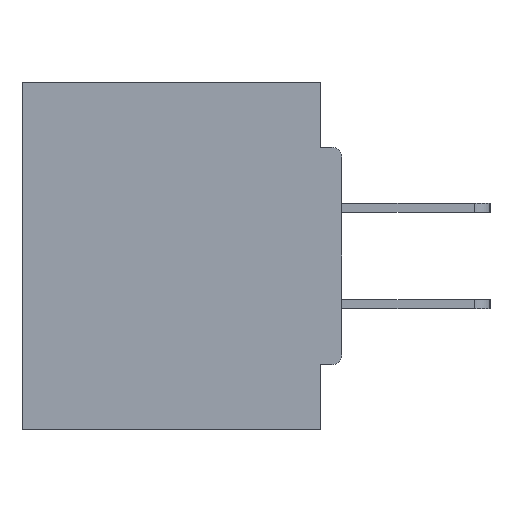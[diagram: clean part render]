
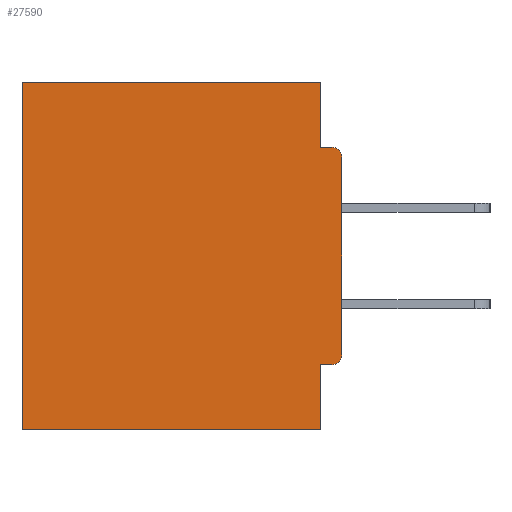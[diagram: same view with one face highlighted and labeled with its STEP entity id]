
A CAD part, left-side view. The second image highlights one B-rep face of the part: STEP entity #27590.
In plain terms, the highlighted planar face has unit normal (-1, 0, 0).
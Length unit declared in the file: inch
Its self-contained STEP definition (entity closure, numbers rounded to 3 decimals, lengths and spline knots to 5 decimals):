
#1164 = CIRCLE ( 'NONE', #3589, 0.015 ) ;
#1298 = CARTESIAN_POINT ( 'NONE',  ( 0.298, 0.031, -0.5 ) ) ;
#2060 = VECTOR ( 'NONE', #28027, 39.37008 ) ;
#2228 = CARTESIAN_POINT ( 'NONE',  ( 0.298, 0.031, -0.5 ) ) ;
#2380 = ORIENTED_EDGE ( 'NONE', *, *, #32719, .F. ) ;
#2655 = EDGE_CURVE ( 'NONE', #3849, #28235, #35394, .T. ) ;
#2682 = CARTESIAN_POINT ( 'NONE',  ( 0.298, 0.015, -0.4065 ) ) ;
#3080 = LINE ( 'NONE', #7466, #18006 ) ;
#3131 = DIRECTION ( 'NONE',  ( 0., 0., -1. ) ) ;
#3264 = CARTESIAN_POINT ( 'NONE',  ( 0.298, 0.015, -0.3915 ) ) ;
#3558 = EDGE_CURVE ( 'NONE', #12391, #12726, #29469, .T. ) ;
#3589 = AXIS2_PLACEMENT_3D ( 'NONE', #14710, #26165, #3684 ) ;
#3684 = DIRECTION ( 'NONE',  ( 0., 0., -1. ) ) ;
#3849 = VERTEX_POINT ( 'NONE', #35695 ) ;
#4348 = CARTESIAN_POINT ( 'NONE',  ( 0.298, 0.46, 0. ) ) ;
#5256 = DIRECTION ( 'NONE',  ( 0., 1., 0. ) ) ;
#6180 = DIRECTION ( 'NONE',  ( 0., 0., -1. ) ) ;
#7466 = CARTESIAN_POINT ( 'NONE',  ( 0.298, 0., -0.5 ) ) ;
#8186 = DIRECTION ( 'NONE',  ( 0., -1., 0. ) ) ;
#8608 = CARTESIAN_POINT ( 'NONE',  ( 0.298, 0.031, -0.5 ) ) ;
#9633 = CARTESIAN_POINT ( 'NONE',  ( 0.298, 0., -0.1085 ) ) ;
#10386 = LINE ( 'NONE', #34632, #16552 ) ;
#10844 = VERTEX_POINT ( 'NONE', #9633 ) ;
#11154 = EDGE_CURVE ( 'NONE', #19791, #27602, #3080, .T. ) ;
#11939 = CARTESIAN_POINT ( 'NONE',  ( 0.298, 0.46, -0.5 ) ) ;
#12018 = DIRECTION ( 'NONE',  ( 0., 1., 0. ) ) ;
#12109 = ORIENTED_EDGE ( 'NONE', *, *, #14190, .F. ) ;
#12391 = VERTEX_POINT ( 'NONE', #35027 ) ;
#12726 = VERTEX_POINT ( 'NONE', #15777 ) ;
#13450 = CARTESIAN_POINT ( 'NONE',  ( 0.298, 0.031, -0.4065 ) ) ;
#13462 = EDGE_CURVE ( 'NONE', #21836, #19791, #30617, .T. ) ;
#13523 = EDGE_CURVE ( 'NONE', #10844, #14720, #10386, .T. ) ;
#14168 = EDGE_CURVE ( 'NONE', #10844, #28235, #1164, .T. ) ;
#14190 = EDGE_CURVE ( 'NONE', #35517, #21836, #15617, .T. ) ;
#14710 = CARTESIAN_POINT ( 'NONE',  ( 0.298, 0.015, -0.1085 ) ) ;
#14720 = VERTEX_POINT ( 'NONE', #17571 ) ;
#15070 = EDGE_CURVE ( 'NONE', #12726, #27602, #18255, .T. ) ;
#15072 = DIRECTION ( 'NONE',  ( 0., 0., -1. ) ) ;
#15617 = LINE ( 'NONE', #23448, #30131 ) ;
#15777 = CARTESIAN_POINT ( 'NONE',  ( 0.298, 0.46, 0. ) ) ;
#15984 = ORIENTED_EDGE ( 'NONE', *, *, #11154, .F. ) ;
#15994 = EDGE_LOOP ( 'NONE', ( #35333, #22785, #2380, #22157, #20107, #15984, #31401, #12109, #30642, #31345 ) ) ;
#16552 = VECTOR ( 'NONE', #15072, 39.37008 ) ;
#17434 = DIRECTION ( 'NONE',  ( 1., 0., 0. ) ) ;
#17571 = CARTESIAN_POINT ( 'NONE',  ( 0.298, 0., -0.3915 ) ) ;
#18006 = VECTOR ( 'NONE', #27127, 39.37008 ) ;
#18083 = DIRECTION ( 'NONE',  ( 0., 0., -1. ) ) ;
#18255 = LINE ( 'NONE', #4348, #35814 ) ;
#18857 = CARTESIAN_POINT ( 'NONE',  ( 0.298, 0., 0. ) ) ;
#19572 = CARTESIAN_POINT ( 'NONE',  ( 0.298, 0., -0.0935 ) ) ;
#19779 = CARTESIAN_POINT ( 'NONE',  ( 0.298, 0.015, -0.0935 ) ) ;
#19791 = VERTEX_POINT ( 'NONE', #1298 ) ;
#20107 = ORIENTED_EDGE ( 'NONE', *, *, #15070, .T. ) ;
#20189 = VECTOR ( 'NONE', #5256, 39.37008 ) ;
#21703 = LINE ( 'NONE', #2228, #34512 ) ;
#21836 = VERTEX_POINT ( 'NONE', #13450 ) ;
#22157 = ORIENTED_EDGE ( 'NONE', *, *, #3558, .T. ) ;
#22785 = ORIENTED_EDGE ( 'NONE', *, *, #2655, .F. ) ;
#23448 = CARTESIAN_POINT ( 'NONE',  ( 0.298, 0., -0.4065 ) ) ;
#24631 = FACE_OUTER_BOUND ( 'NONE', #15994, .T. ) ;
#24753 = CIRCLE ( 'NONE', #32007, 0.015 ) ;
#25465 = PLANE ( 'NONE',  #34711 ) ;
#26165 = DIRECTION ( 'NONE',  ( -1., 0., 0. ) ) ;
#27127 = DIRECTION ( 'NONE',  ( 0., 1., 0. ) ) ;
#27299 = DIRECTION ( 'NONE',  ( 0., 0., -1. ) ) ;
#27590 = ADVANCED_FACE ( 'NONE', ( #24631 ), #25465, .F. ) ;
#27602 = VERTEX_POINT ( 'NONE', #11939 ) ;
#28027 = DIRECTION ( 'NONE',  ( 0., 0., -1. ) ) ;
#28235 = VERTEX_POINT ( 'NONE', #19779 ) ;
#29296 = VECTOR ( 'NONE', #8186, 39.37008 ) ;
#29469 = LINE ( 'NONE', #18857, #20189 ) ;
#30131 = VECTOR ( 'NONE', #12018, 39.37008 ) ;
#30617 = LINE ( 'NONE', #8608, #2060 ) ;
#30642 = ORIENTED_EDGE ( 'NONE', *, *, #33544, .T. ) ;
#31345 = ORIENTED_EDGE ( 'NONE', *, *, #13523, .F. ) ;
#31401 = ORIENTED_EDGE ( 'NONE', *, *, #13462, .F. ) ;
#32007 = AXIS2_PLACEMENT_3D ( 'NONE', #3264, #34209, #3131 ) ;
#32719 = EDGE_CURVE ( 'NONE', #12391, #3849, #21703, .T. ) ;
#33544 = EDGE_CURVE ( 'NONE', #35517, #14720, #24753, .T. ) ;
#34053 = CARTESIAN_POINT ( 'NONE',  ( 0.298, 0., 0. ) ) ;
#34209 = DIRECTION ( 'NONE',  ( -1., 0., 0. ) ) ;
#34512 = VECTOR ( 'NONE', #27299, 39.37008 ) ;
#34632 = CARTESIAN_POINT ( 'NONE',  ( 0.298, 0., 0. ) ) ;
#34711 = AXIS2_PLACEMENT_3D ( 'NONE', #34053, #17434, #6180 ) ;
#35027 = CARTESIAN_POINT ( 'NONE',  ( 0.298, 0.031, 0. ) ) ;
#35333 = ORIENTED_EDGE ( 'NONE', *, *, #14168, .T. ) ;
#35394 = LINE ( 'NONE', #19572, #29296 ) ;
#35517 = VERTEX_POINT ( 'NONE', #2682 ) ;
#35695 = CARTESIAN_POINT ( 'NONE',  ( 0.298, 0.031, -0.0935 ) ) ;
#35814 = VECTOR ( 'NONE', #18083, 39.37008 ) ;
